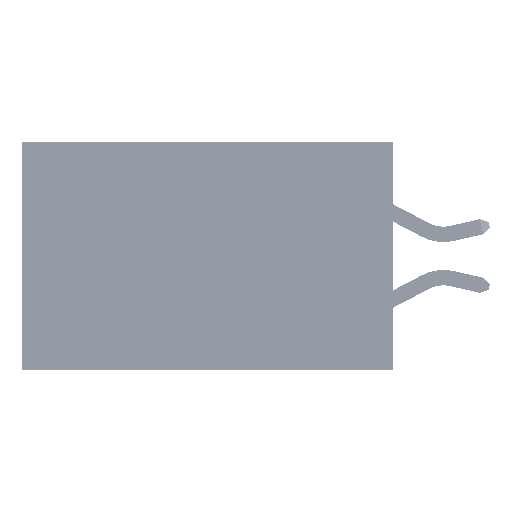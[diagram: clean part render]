
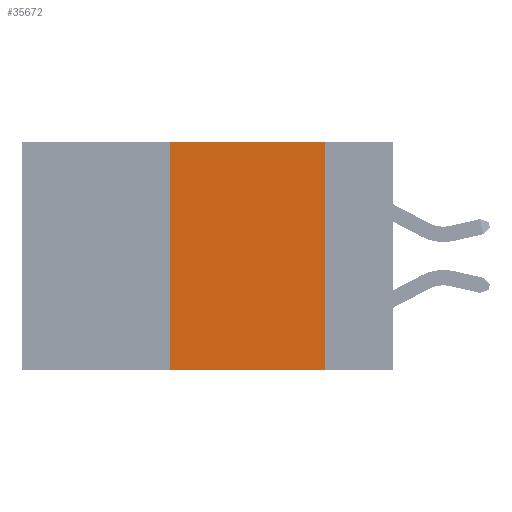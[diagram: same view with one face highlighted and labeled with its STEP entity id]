
A CAD part, left-side view. The second image highlights one B-rep face of the part: STEP entity #35672.
In plain terms, the highlighted planar face has unit normal (-1, 0, 0).
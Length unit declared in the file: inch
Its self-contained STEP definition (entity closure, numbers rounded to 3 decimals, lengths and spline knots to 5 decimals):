
#867 = FACE_OUTER_BOUND ( 'NONE', #2554, .T. ) ;
#1691 = LINE ( 'NONE', #2639, #8545 ) ;
#1956 = VERTEX_POINT ( 'NONE', #2384 ) ;
#2000 = DIRECTION ( 'NONE',  ( 1., 0., 0. ) ) ;
#2076 = DIRECTION ( 'NONE',  ( 0., -1., 0. ) ) ;
#2308 = DIRECTION ( 'NONE',  ( 0., -1., 0. ) ) ;
#2384 = CARTESIAN_POINT ( 'NONE',  ( 0., 0.36, 0. ) ) ;
#2554 = EDGE_LOOP ( 'NONE', ( #30341, #34948, #16743, #11216 ) ) ;
#2639 = CARTESIAN_POINT ( 'NONE',  ( 0., 0.6, 0. ) ) ;
#3307 = AXIS2_PLACEMENT_3D ( 'NONE', #34483, #2000, #9311 ) ;
#7082 = VERTEX_POINT ( 'NONE', #35067 ) ;
#8545 = VECTOR ( 'NONE', #2308, 39.37008 ) ;
#9152 = PLANE ( 'NONE',  #3307 ) ;
#9304 = CARTESIAN_POINT ( 'NONE',  ( 0., 0.11, 0. ) ) ;
#9311 = DIRECTION ( 'NONE',  ( 0., 0., -1. ) ) ;
#9734 = EDGE_CURVE ( 'NONE', #44145, #34813, #45698, .T. ) ;
#10105 = DIRECTION ( 'NONE',  ( 0., 0., -1. ) ) ;
#11216 = ORIENTED_EDGE ( 'NONE', *, *, #12274, .T. ) ;
#12274 = EDGE_CURVE ( 'NONE', #7082, #34813, #39736, .T. ) ;
#16675 = EDGE_CURVE ( 'NONE', #1956, #44145, #1691, .T. ) ;
#16743 = ORIENTED_EDGE ( 'NONE', *, *, #25182, .F. ) ;
#16768 = VECTOR ( 'NONE', #10105, 39.37008 ) ;
#23040 = LINE ( 'NONE', #46220, #41156 ) ;
#23826 = CARTESIAN_POINT ( 'NONE',  ( 0., 0.6, -0.37 ) ) ;
#25182 = EDGE_CURVE ( 'NONE', #7082, #1956, #23040, .T. ) ;
#30341 = ORIENTED_EDGE ( 'NONE', *, *, #9734, .F. ) ;
#31493 = CARTESIAN_POINT ( 'NONE',  ( 0., 0.11, 0. ) ) ;
#34483 = CARTESIAN_POINT ( 'NONE',  ( 0., 0.6, 0. ) ) ;
#34813 = VERTEX_POINT ( 'NONE', #40333 ) ;
#34948 = ORIENTED_EDGE ( 'NONE', *, *, #16675, .F. ) ;
#35067 = CARTESIAN_POINT ( 'NONE',  ( 0., 0.36, -0.37 ) ) ;
#35672 = ADVANCED_FACE ( 'NONE', ( #867 ), #9152, .F. ) ;
#38041 = VECTOR ( 'NONE', #2076, 39.37008 ) ;
#39037 = DIRECTION ( 'NONE',  ( 0., 0., 1. ) ) ;
#39736 = LINE ( 'NONE', #23826, #38041 ) ;
#40333 = CARTESIAN_POINT ( 'NONE',  ( 0., 0.11, -0.37 ) ) ;
#41156 = VECTOR ( 'NONE', #39037, 39.37008 ) ;
#44145 = VERTEX_POINT ( 'NONE', #9304 ) ;
#45698 = LINE ( 'NONE', #31493, #16768 ) ;
#46220 = CARTESIAN_POINT ( 'NONE',  ( 0., 0.36, 0. ) ) ;
